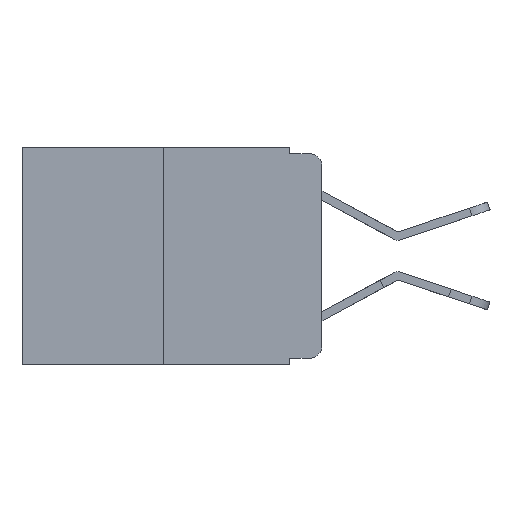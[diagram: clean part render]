
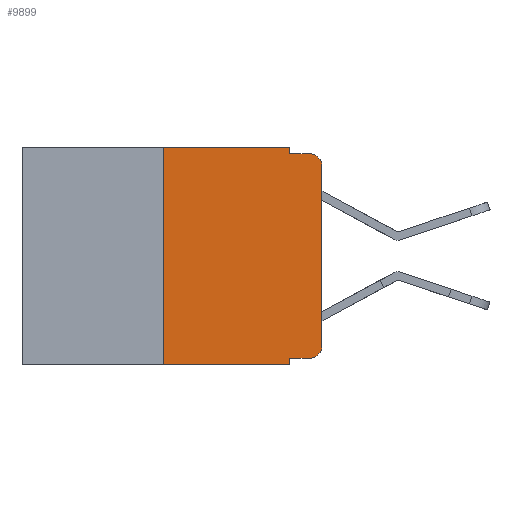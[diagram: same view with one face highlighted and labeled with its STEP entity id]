
A CAD part, left-side view. The second image highlights one B-rep face of the part: STEP entity #9899.
In plain terms, the highlighted planar face has unit normal (-1, 0, 0).
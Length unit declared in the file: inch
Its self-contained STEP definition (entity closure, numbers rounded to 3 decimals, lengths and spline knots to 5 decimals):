
#90 = CARTESIAN_POINT ( 'NONE',  ( 0., 0.051, -0.01 ) ) ;
#596 = ORIENTED_EDGE ( 'NONE', *, *, #22740, .T. ) ;
#825 = CARTESIAN_POINT ( 'NONE',  ( 0., 0.02, -0.01 ) ) ;
#1119 = LINE ( 'NONE', #6072, #12593 ) ;
#1157 = DIRECTION ( 'NONE',  ( 0., 0., -1. ) ) ;
#1406 = ORIENTED_EDGE ( 'NONE', *, *, #21114, .F. ) ;
#1604 = DIRECTION ( 'NONE',  ( 0., -1., 0. ) ) ;
#2200 = EDGE_CURVE ( 'NONE', #5945, #20305, #11079, .T. ) ;
#2616 = DIRECTION ( 'NONE',  ( 0., -1., 0. ) ) ;
#2651 = ORIENTED_EDGE ( 'NONE', *, *, #15159, .T. ) ;
#3302 = LINE ( 'NONE', #21352, #8145 ) ;
#3449 = ORIENTED_EDGE ( 'NONE', *, *, #4503, .F. ) ;
#3502 = CIRCLE ( 'NONE', #23191, 0.02 ) ;
#3545 = CARTESIAN_POINT ( 'NONE',  ( 0., 0.051, 0. ) ) ;
#4503 = EDGE_CURVE ( 'NONE', #11487, #7344, #25946, .T. ) ;
#4710 = AXIS2_PLACEMENT_3D ( 'NONE', #19649, #15650, #11624 ) ;
#4880 = CARTESIAN_POINT ( 'NONE',  ( 0., 0.051, 0. ) ) ;
#5779 = EDGE_LOOP ( 'NONE', ( #2651, #22263, #7201, #11493, #3449, #1406, #596, #25294, #16639, #19146 ) ) ;
#5945 = VERTEX_POINT ( 'NONE', #15041 ) ;
#6072 = CARTESIAN_POINT ( 'NONE',  ( 0., 0.051, -0.333 ) ) ;
#6487 = CARTESIAN_POINT ( 'NONE',  ( 0., 0.473, 0. ) ) ;
#7138 = VECTOR ( 'NONE', #2616, 39.37008 ) ;
#7201 = ORIENTED_EDGE ( 'NONE', *, *, #25476, .F. ) ;
#7344 = VERTEX_POINT ( 'NONE', #3545 ) ;
#7751 = CARTESIAN_POINT ( 'NONE',  ( 0., 0., -0.03 ) ) ;
#7885 = DIRECTION ( 'NONE',  ( 0., 0., -1. ) ) ;
#7988 = VECTOR ( 'NONE', #1157, 39.37008 ) ;
#8145 = VECTOR ( 'NONE', #25348, 39.37008 ) ;
#8214 = VECTOR ( 'NONE', #21698, 39.37008 ) ;
#9589 = DIRECTION ( 'NONE',  ( 0., 0., -1. ) ) ;
#9801 = VERTEX_POINT ( 'NONE', #825 ) ;
#9899 = ADVANCED_FACE ( 'NONE', ( #10864 ), #13614, .F. ) ;
#9924 = CARTESIAN_POINT ( 'NONE',  ( 0., 0., 0. ) ) ;
#9967 = DIRECTION ( 'NONE',  ( 0., 0., -1. ) ) ;
#10454 = VECTOR ( 'NONE', #9589, 39.37008 ) ;
#10698 = VERTEX_POINT ( 'NONE', #22533 ) ;
#10767 = CARTESIAN_POINT ( 'NONE',  ( 0., 0.051, -0.343 ) ) ;
#10864 = FACE_OUTER_BOUND ( 'NONE', #5779, .T. ) ;
#11079 = LINE ( 'NONE', #4880, #10454 ) ;
#11213 = EDGE_CURVE ( 'NONE', #17950, #9801, #3502, .T. ) ;
#11288 = VERTEX_POINT ( 'NONE', #18271 ) ;
#11363 = CARTESIAN_POINT ( 'NONE',  ( 0., 0.25, 0. ) ) ;
#11380 = LINE ( 'NONE', #11363, #8214 ) ;
#11487 = VERTEX_POINT ( 'NONE', #12811 ) ;
#11493 = ORIENTED_EDGE ( 'NONE', *, *, #19809, .F. ) ;
#11563 = VERTEX_POINT ( 'NONE', #15203 ) ;
#11618 = DIRECTION ( 'NONE',  ( 0., 0., 1. ) ) ;
#11624 = DIRECTION ( 'NONE',  ( 0., 0., -1. ) ) ;
#11880 = DIRECTION ( 'NONE',  ( -1., 0., 0. ) ) ;
#12415 = DIRECTION ( 'NONE',  ( 0., -1., 0. ) ) ;
#12593 = VECTOR ( 'NONE', #1604, 39.37008 ) ;
#12811 = CARTESIAN_POINT ( 'NONE',  ( 0., 0.25, 0. ) ) ;
#13368 = VERTEX_POINT ( 'NONE', #18145 ) ;
#13614 = PLANE ( 'NONE',  #4710 ) ;
#13758 = LINE ( 'NONE', #90, #16926 ) ;
#13903 = EDGE_CURVE ( 'NONE', #5945, #11563, #1119, .T. ) ;
#14105 = DIRECTION ( 'NONE',  ( -1., 0., 0. ) ) ;
#15041 = CARTESIAN_POINT ( 'NONE',  ( 0., 0.051, -0.333 ) ) ;
#15159 = EDGE_CURVE ( 'NONE', #10698, #17950, #24132, .T. ) ;
#15203 = CARTESIAN_POINT ( 'NONE',  ( 0., 0.02, -0.333 ) ) ;
#15650 = DIRECTION ( 'NONE',  ( 1., 0., 0. ) ) ;
#16270 = LINE ( 'NONE', #19341, #7988 ) ;
#16639 = ORIENTED_EDGE ( 'NONE', *, *, #13903, .T. ) ;
#16770 = EDGE_CURVE ( 'NONE', #11563, #10698, #23746, .T. ) ;
#16926 = VECTOR ( 'NONE', #12415, 39.37008 ) ;
#17950 = VERTEX_POINT ( 'NONE', #7751 ) ;
#18050 = CARTESIAN_POINT ( 'NONE',  ( 0., 0.02, -0.313 ) ) ;
#18145 = CARTESIAN_POINT ( 'NONE',  ( 0., 0.25, -0.343 ) ) ;
#18271 = CARTESIAN_POINT ( 'NONE',  ( 0., 0.051, -0.01 ) ) ;
#19146 = ORIENTED_EDGE ( 'NONE', *, *, #16770, .T. ) ;
#19341 = CARTESIAN_POINT ( 'NONE',  ( 0., 0.051, 0. ) ) ;
#19649 = CARTESIAN_POINT ( 'NONE',  ( 0., 0.473, 0. ) ) ;
#19809 = EDGE_CURVE ( 'NONE', #7344, #11288, #16270, .T. ) ;
#20193 = CARTESIAN_POINT ( 'NONE',  ( 0., 0.02, -0.03 ) ) ;
#20305 = VERTEX_POINT ( 'NONE', #10767 ) ;
#21114 = EDGE_CURVE ( 'NONE', #13368, #11487, #11380, .T. ) ;
#21352 = CARTESIAN_POINT ( 'NONE',  ( 0., 0.473, -0.343 ) ) ;
#21561 = VECTOR ( 'NONE', #11618, 39.37008 ) ;
#21698 = DIRECTION ( 'NONE',  ( 0., 0., 1. ) ) ;
#22263 = ORIENTED_EDGE ( 'NONE', *, *, #11213, .T. ) ;
#22533 = CARTESIAN_POINT ( 'NONE',  ( 0., 0., -0.313 ) ) ;
#22740 = EDGE_CURVE ( 'NONE', #13368, #20305, #3302, .T. ) ;
#23191 = AXIS2_PLACEMENT_3D ( 'NONE', #20193, #14105, #9967 ) ;
#23746 = CIRCLE ( 'NONE', #25336, 0.02 ) ;
#24132 = LINE ( 'NONE', #9924, #21561 ) ;
#25294 = ORIENTED_EDGE ( 'NONE', *, *, #2200, .F. ) ;
#25336 = AXIS2_PLACEMENT_3D ( 'NONE', #18050, #11880, #7885 ) ;
#25348 = DIRECTION ( 'NONE',  ( 0., -1., 0. ) ) ;
#25476 = EDGE_CURVE ( 'NONE', #11288, #9801, #13758, .T. ) ;
#25946 = LINE ( 'NONE', #6487, #7138 ) ;
